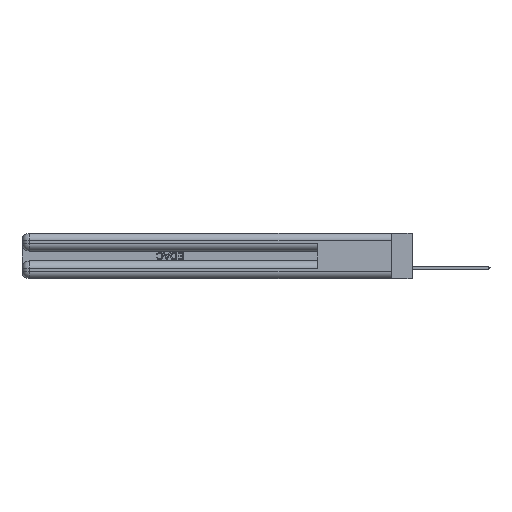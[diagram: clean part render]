
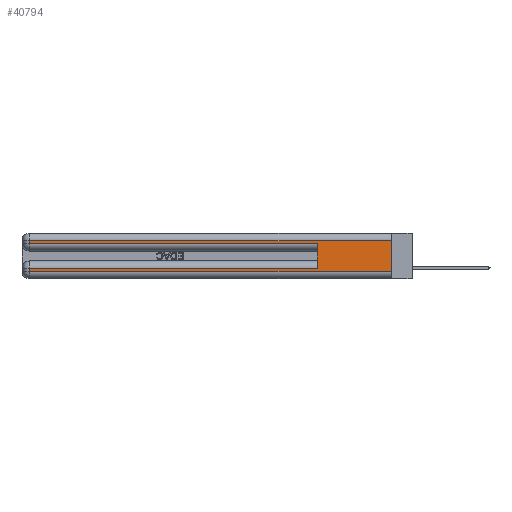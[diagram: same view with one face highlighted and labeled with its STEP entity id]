
A CAD part, left-side view. The second image highlights one B-rep face of the part: STEP entity #40794.
In plain terms, the highlighted planar face has unit normal (-1, 0, 0).
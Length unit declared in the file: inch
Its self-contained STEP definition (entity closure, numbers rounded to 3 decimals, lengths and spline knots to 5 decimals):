
#489 = ORIENTED_EDGE ( 'NONE', *, *, #50290, .T. ) ;
#562 = PLANE ( 'NONE',  #20839 ) ;
#1144 = ORIENTED_EDGE ( 'NONE', *, *, #14366, .F. ) ;
#1873 = CARTESIAN_POINT ( 'NONE',  ( 0., 0., 0.37 ) ) ;
#2407 = VECTOR ( 'NONE', #4579, 39.37008 ) ;
#2857 = CARTESIAN_POINT ( 'NONE',  ( 0., 2.94, 0.06 ) ) ;
#4336 = DIRECTION ( 'NONE',  ( 1., 0., 0. ) ) ;
#4380 = CARTESIAN_POINT ( 'NONE',  ( 0., 0.6, 0.145 ) ) ;
#4579 = DIRECTION ( 'NONE',  ( 0., -1., 0. ) ) ;
#5129 = CARTESIAN_POINT ( 'NONE',  ( 0., 2.94, 0.37 ) ) ;
#6775 = LINE ( 'NONE', #1873, #43380 ) ;
#7522 = EDGE_CURVE ( 'NONE', #41881, #37679, #27951, .T. ) ;
#8238 = CARTESIAN_POINT ( 'NONE',  ( 0., 2.94, 0.285 ) ) ;
#8505 = CARTESIAN_POINT ( 'NONE',  ( 0., 2.94, 0.31 ) ) ;
#11745 = CARTESIAN_POINT ( 'NONE',  ( 0., 0., 0.31 ) ) ;
#12945 = EDGE_CURVE ( 'NONE', #42258, #17054, #28582, .T. ) ;
#13966 = CARTESIAN_POINT ( 'NONE',  ( 0., 0., 0.06 ) ) ;
#14366 = EDGE_CURVE ( 'NONE', #22823, #37679, #6775, .T. ) ;
#15633 = CARTESIAN_POINT ( 'NONE',  ( 0., 2.94, 0.37 ) ) ;
#17054 = VERTEX_POINT ( 'NONE', #44027 ) ;
#17694 = CARTESIAN_POINT ( 'NONE',  ( 0., 0., 0.085 ) ) ;
#17973 = LINE ( 'NONE', #4380, #40018 ) ;
#18429 = VECTOR ( 'NONE', #28588, 39.37008 ) ;
#20192 = FACE_OUTER_BOUND ( 'NONE', #39770, .T. ) ;
#20721 = VERTEX_POINT ( 'NONE', #8505 ) ;
#20839 = AXIS2_PLACEMENT_3D ( 'NONE', #31241, #4336, #31065 ) ;
#21782 = DIRECTION ( 'NONE',  ( 0., 0., -1. ) ) ;
#21813 = VECTOR ( 'NONE', #41388, 39.37008 ) ;
#22137 = LINE ( 'NONE', #17694, #28276 ) ;
#22823 = VERTEX_POINT ( 'NONE', #11745 ) ;
#23902 = EDGE_CURVE ( 'NONE', #44106, #41881, #47402, .T. ) ;
#24623 = EDGE_CURVE ( 'NONE', #36706, #17054, #17973, .T. ) ;
#25889 = LINE ( 'NONE', #30754, #47882 ) ;
#26773 = ORIENTED_EDGE ( 'NONE', *, *, #12945, .T. ) ;
#27951 = LINE ( 'NONE', #13966, #21813 ) ;
#28012 = ORIENTED_EDGE ( 'NONE', *, *, #7522, .T. ) ;
#28276 = VECTOR ( 'NONE', #29133, 39.37008 ) ;
#28582 = LINE ( 'NONE', #47831, #2407 ) ;
#28588 = DIRECTION ( 'NONE',  ( 0., 0., -1. ) ) ;
#29133 = DIRECTION ( 'NONE',  ( 0., 1., 0. ) ) ;
#30754 = CARTESIAN_POINT ( 'NONE',  ( 0., 0., 0.31 ) ) ;
#31065 = DIRECTION ( 'NONE',  ( 0., 0., -1. ) ) ;
#31241 = CARTESIAN_POINT ( 'NONE',  ( 0., 0., 0.37 ) ) ;
#34201 = DIRECTION ( 'NONE',  ( 0., 1., 0. ) ) ;
#35290 = ORIENTED_EDGE ( 'NONE', *, *, #43224, .T. ) ;
#36706 = VERTEX_POINT ( 'NONE', #48521 ) ;
#36783 = LINE ( 'NONE', #5129, #18429 ) ;
#37679 = VERTEX_POINT ( 'NONE', #43869 ) ;
#37840 = ORIENTED_EDGE ( 'NONE', *, *, #24623, .F. ) ;
#38888 = VECTOR ( 'NONE', #47362, 39.37008 ) ;
#39200 = EDGE_CURVE ( 'NONE', #36706, #44106, #22137, .T. ) ;
#39770 = EDGE_LOOP ( 'NONE', ( #1144, #35290, #489, #26773, #37840, #45700, #44242, #28012 ) ) ;
#40018 = VECTOR ( 'NONE', #47297, 39.37008 ) ;
#40282 = CARTESIAN_POINT ( 'NONE',  ( 0., 2.94, 0.085 ) ) ;
#40794 = ADVANCED_FACE ( 'NONE', ( #20192 ), #562, .F. ) ;
#41388 = DIRECTION ( 'NONE',  ( 0., -1., 0. ) ) ;
#41881 = VERTEX_POINT ( 'NONE', #2857 ) ;
#42258 = VERTEX_POINT ( 'NONE', #8238 ) ;
#43224 = EDGE_CURVE ( 'NONE', #22823, #20721, #25889, .T. ) ;
#43380 = VECTOR ( 'NONE', #21782, 39.37008 ) ;
#43869 = CARTESIAN_POINT ( 'NONE',  ( 0., 0., 0.06 ) ) ;
#44027 = CARTESIAN_POINT ( 'NONE',  ( 0., 0.6, 0.285 ) ) ;
#44106 = VERTEX_POINT ( 'NONE', #40282 ) ;
#44242 = ORIENTED_EDGE ( 'NONE', *, *, #23902, .T. ) ;
#45700 = ORIENTED_EDGE ( 'NONE', *, *, #39200, .T. ) ;
#47297 = DIRECTION ( 'NONE',  ( 0., 0., 1. ) ) ;
#47362 = DIRECTION ( 'NONE',  ( 0., 0., -1. ) ) ;
#47402 = LINE ( 'NONE', #15633, #38888 ) ;
#47831 = CARTESIAN_POINT ( 'NONE',  ( 0., 0., 0.285 ) ) ;
#47882 = VECTOR ( 'NONE', #34201, 39.37008 ) ;
#48521 = CARTESIAN_POINT ( 'NONE',  ( 0., 0.6, 0.085 ) ) ;
#50290 = EDGE_CURVE ( 'NONE', #20721, #42258, #36783, .T. ) ;
